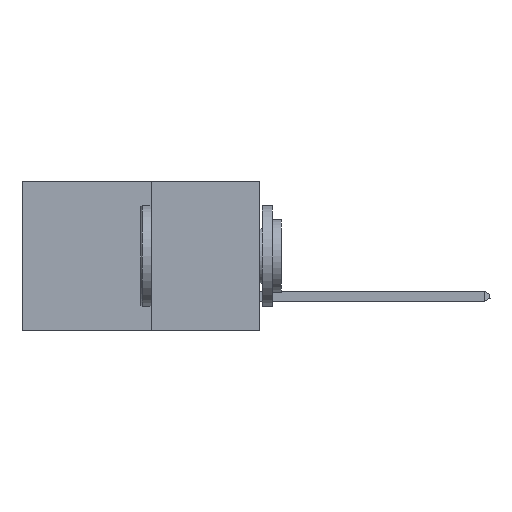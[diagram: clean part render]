
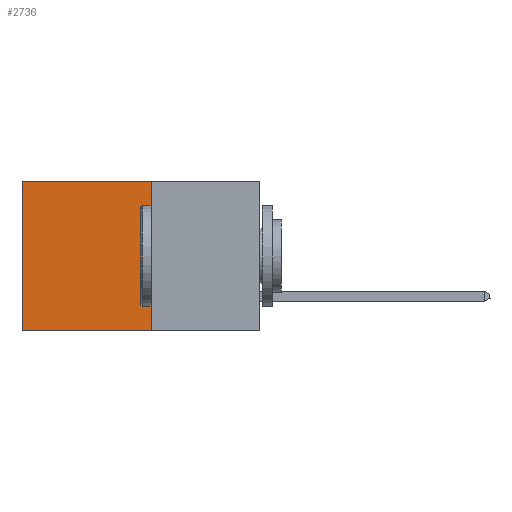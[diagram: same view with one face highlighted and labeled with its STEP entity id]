
A CAD part, left-side view. The second image highlights one B-rep face of the part: STEP entity #2736.
In plain terms, the highlighted planar face has unit normal (-1, 0, 0).
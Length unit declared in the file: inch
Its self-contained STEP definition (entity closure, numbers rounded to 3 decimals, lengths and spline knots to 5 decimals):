
#16 = LINE ( 'NONE', #13104, #3261 ) ;
#304 = VERTEX_POINT ( 'NONE', #5841 ) ;
#657 = ORIENTED_EDGE ( 'NONE', *, *, #15513, .T. ) ;
#684 = VECTOR ( 'NONE', #10124, 39.37008 ) ;
#1170 = ORIENTED_EDGE ( 'NONE', *, *, #10839, .F. ) ;
#1818 = VECTOR ( 'NONE', #7421, 39.37008 ) ;
#2196 = CARTESIAN_POINT ( 'NONE',  ( 0.277, 0.27, 0. ) ) ;
#2693 = AXIS2_PLACEMENT_3D ( 'NONE', #5452, #5232, #5116 ) ;
#2736 = ADVANCED_FACE ( 'NONE', ( #10202 ), #6780, .F. ) ;
#2763 = EDGE_CURVE ( 'NONE', #8897, #304, #16, .T. ) ;
#3028 = ORIENTED_EDGE ( 'NONE', *, *, #10198, .T. ) ;
#3261 = VECTOR ( 'NONE', #12285, 39.37008 ) ;
#3891 = LINE ( 'NONE', #12778, #684 ) ;
#5018 = CARTESIAN_POINT ( 'NONE',  ( 0.277, 0.59, 0. ) ) ;
#5116 = DIRECTION ( 'NONE',  ( 0., 0., -1. ) ) ;
#5232 = DIRECTION ( 'NONE',  ( 1., 0., 0. ) ) ;
#5452 = CARTESIAN_POINT ( 'NONE',  ( 0.277, 0.27, -0.37 ) ) ;
#5509 = EDGE_LOOP ( 'NONE', ( #657, #1170, #15935, #3028 ) ) ;
#5841 = CARTESIAN_POINT ( 'NONE',  ( 0.277, 0.27, -0.37 ) ) ;
#6543 = VERTEX_POINT ( 'NONE', #5018 ) ;
#6780 = PLANE ( 'NONE',  #2693 ) ;
#7421 = DIRECTION ( 'NONE',  ( 0., 0., -1. ) ) ;
#8322 = LINE ( 'NONE', #13991, #14861 ) ;
#8579 = VERTEX_POINT ( 'NONE', #14668 ) ;
#8897 = VERTEX_POINT ( 'NONE', #2196 ) ;
#10124 = DIRECTION ( 'NONE',  ( 0., 1., 0. ) ) ;
#10198 = EDGE_CURVE ( 'NONE', #8897, #6543, #3891, .T. ) ;
#10202 = FACE_OUTER_BOUND ( 'NONE', #5509, .T. ) ;
#10839 = EDGE_CURVE ( 'NONE', #304, #8579, #8322, .T. ) ;
#11911 = LINE ( 'NONE', #15230, #1818 ) ;
#12285 = DIRECTION ( 'NONE',  ( 0., 0., -1. ) ) ;
#12778 = CARTESIAN_POINT ( 'NONE',  ( 0.277, 0.27, 0. ) ) ;
#13104 = CARTESIAN_POINT ( 'NONE',  ( 0.277, 0.27, -0.37 ) ) ;
#13991 = CARTESIAN_POINT ( 'NONE',  ( 0.277, 0.27, -0.37 ) ) ;
#14668 = CARTESIAN_POINT ( 'NONE',  ( 0.277, 0.59, -0.37 ) ) ;
#14861 = VECTOR ( 'NONE', #15261, 39.37008 ) ;
#15230 = CARTESIAN_POINT ( 'NONE',  ( 0.277, 0.59, -0.37 ) ) ;
#15261 = DIRECTION ( 'NONE',  ( 0., 1., 0. ) ) ;
#15513 = EDGE_CURVE ( 'NONE', #6543, #8579, #11911, .T. ) ;
#15935 = ORIENTED_EDGE ( 'NONE', *, *, #2763, .F. ) ;
